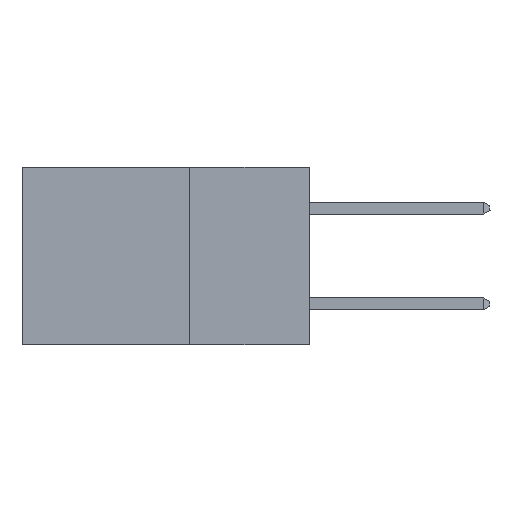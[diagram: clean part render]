
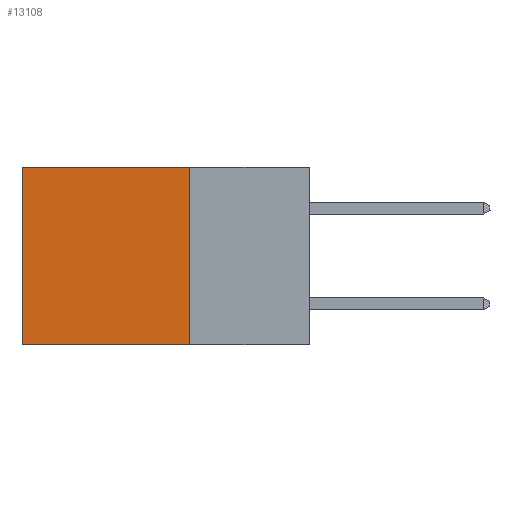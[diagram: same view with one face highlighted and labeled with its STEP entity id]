
A CAD part, left-side view. The second image highlights one B-rep face of the part: STEP entity #13108.
In plain terms, the highlighted planar face has unit normal (-1, 0, 0).
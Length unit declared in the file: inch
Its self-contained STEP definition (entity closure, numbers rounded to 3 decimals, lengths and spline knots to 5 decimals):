
#442 = EDGE_CURVE ( 'NONE', #11122, #3557, #19057, .T. ) ;
#1662 = CARTESIAN_POINT ( 'NONE',  ( 0.2875, 0.25, -0.37 ) ) ;
#2016 = ORIENTED_EDGE ( 'NONE', *, *, #2349, .T. ) ;
#2265 = ORIENTED_EDGE ( 'NONE', *, *, #13224, .F. ) ;
#2349 = EDGE_CURVE ( 'NONE', #3557, #7800, #11374, .T. ) ;
#2643 = PLANE ( 'NONE',  #14493 ) ;
#2756 = CARTESIAN_POINT ( 'NONE',  ( 0.2875, 0.6, -0.37 ) ) ;
#3557 = VERTEX_POINT ( 'NONE', #24625 ) ;
#4583 = CARTESIAN_POINT ( 'NONE',  ( 0.2875, 0.25, 0. ) ) ;
#5767 = DIRECTION ( 'NONE',  ( 0., 0., -1. ) ) ;
#7800 = VERTEX_POINT ( 'NONE', #2756 ) ;
#10062 = VERTEX_POINT ( 'NONE', #1662 ) ;
#10794 = FACE_OUTER_BOUND ( 'NONE', #20581, .T. ) ;
#11122 = VERTEX_POINT ( 'NONE', #13310 ) ;
#11374 = LINE ( 'NONE', #23189, #23973 ) ;
#11652 = VECTOR ( 'NONE', #15283, 39.37008 ) ;
#13082 = CARTESIAN_POINT ( 'NONE',  ( 0.2875, 0.25, 0. ) ) ;
#13108 = ADVANCED_FACE ( 'NONE', ( #10794 ), #2643, .F. ) ;
#13224 = EDGE_CURVE ( 'NONE', #10062, #7800, #17513, .T. ) ;
#13310 = CARTESIAN_POINT ( 'NONE',  ( 0.2875, 0.25, 0. ) ) ;
#14493 = AXIS2_PLACEMENT_3D ( 'NONE', #4583, #18323, #16629 ) ;
#15283 = DIRECTION ( 'NONE',  ( 0., 1., 0. ) ) ;
#15611 = CARTESIAN_POINT ( 'NONE',  ( 0.2875, 0.25, 0. ) ) ;
#16629 = DIRECTION ( 'NONE',  ( 0., 0., -1. ) ) ;
#16757 = ORIENTED_EDGE ( 'NONE', *, *, #24914, .F. ) ;
#17513 = LINE ( 'NONE', #22732, #24831 ) ;
#17564 = LINE ( 'NONE', #15611, #25004 ) ;
#18323 = DIRECTION ( 'NONE',  ( 1., 0., 0. ) ) ;
#19057 = LINE ( 'NONE', #13082, #11652 ) ;
#20581 = EDGE_LOOP ( 'NONE', ( #2016, #2265, #16757, #21307 ) ) ;
#21307 = ORIENTED_EDGE ( 'NONE', *, *, #442, .T. ) ;
#22732 = CARTESIAN_POINT ( 'NONE',  ( 0.2875, 0.25, -0.37 ) ) ;
#23189 = CARTESIAN_POINT ( 'NONE',  ( 0.2875, 0.6, 0. ) ) ;
#23314 = DIRECTION ( 'NONE',  ( 0., 0., -1. ) ) ;
#23475 = DIRECTION ( 'NONE',  ( 0., 1., 0. ) ) ;
#23973 = VECTOR ( 'NONE', #23314, 39.37008 ) ;
#24625 = CARTESIAN_POINT ( 'NONE',  ( 0.2875, 0.6, 0. ) ) ;
#24831 = VECTOR ( 'NONE', #23475, 39.37008 ) ;
#24914 = EDGE_CURVE ( 'NONE', #11122, #10062, #17564, .T. ) ;
#25004 = VECTOR ( 'NONE', #5767, 39.37008 ) ;
